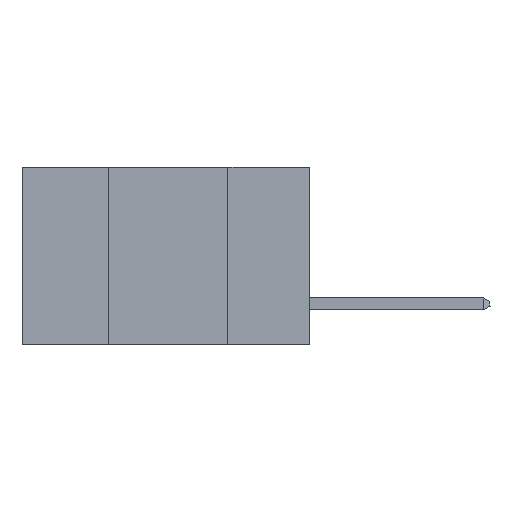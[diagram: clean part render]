
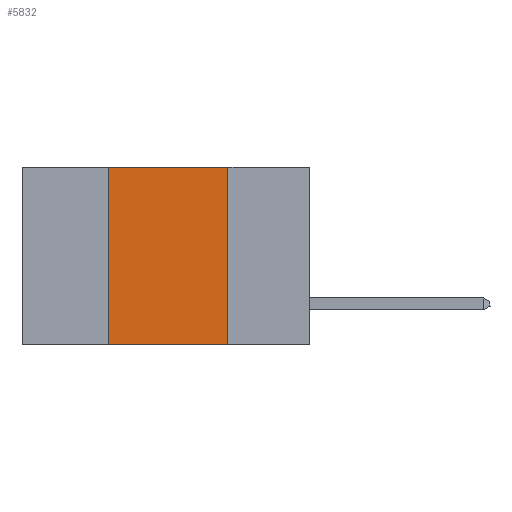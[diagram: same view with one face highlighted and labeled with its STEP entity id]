
A CAD part, left-side view. The second image highlights one B-rep face of the part: STEP entity #5832.
In plain terms, the highlighted planar face has unit normal (-1, 0, 0).
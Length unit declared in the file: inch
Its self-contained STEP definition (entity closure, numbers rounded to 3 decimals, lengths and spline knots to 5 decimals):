
#355 = DIRECTION ( 'NONE',  ( 0., -1., 0. ) ) ;
#1837 = DIRECTION ( 'NONE',  ( 0., -1., 0. ) ) ;
#2146 = ORIENTED_EDGE ( 'NONE', *, *, #18945, .F. ) ;
#2621 = VERTEX_POINT ( 'NONE', #10807 ) ;
#4374 = LINE ( 'NONE', #6501, #4651 ) ;
#4651 = VECTOR ( 'NONE', #21407, 39.37008 ) ;
#5076 = VERTEX_POINT ( 'NONE', #5207 ) ;
#5207 = CARTESIAN_POINT ( 'NONE',  ( 0., 0.42, 0. ) ) ;
#5384 = VECTOR ( 'NONE', #1837, 39.37008 ) ;
#5832 = ADVANCED_FACE ( 'NONE', ( #17424 ), #8938, .F. ) ;
#6370 = EDGE_CURVE ( 'NONE', #14879, #2621, #12262, .T. ) ;
#6501 = CARTESIAN_POINT ( 'NONE',  ( 0., 0.17, 0. ) ) ;
#7292 = CARTESIAN_POINT ( 'NONE',  ( 0., 0.42, 0. ) ) ;
#7399 = CARTESIAN_POINT ( 'NONE',  ( 0., 0.6, 0. ) ) ;
#7805 = EDGE_CURVE ( 'NONE', #16704, #2621, #4374, .T. ) ;
#8421 = LINE ( 'NONE', #7292, #16571 ) ;
#8685 = LINE ( 'NONE', #22218, #18203 ) ;
#8938 = PLANE ( 'NONE',  #21732 ) ;
#10503 = CARTESIAN_POINT ( 'NONE',  ( 0., 0.6, -0.37 ) ) ;
#10643 = DIRECTION ( 'NONE',  ( 0., 0., -1. ) ) ;
#10807 = CARTESIAN_POINT ( 'NONE',  ( 0., 0.17, -0.37 ) ) ;
#11539 = CARTESIAN_POINT ( 'NONE',  ( 0., 0.42, -0.37 ) ) ;
#11978 = EDGE_LOOP ( 'NONE', ( #21581, #2146, #12144, #13847 ) ) ;
#12144 = ORIENTED_EDGE ( 'NONE', *, *, #21015, .F. ) ;
#12262 = LINE ( 'NONE', #10503, #5384 ) ;
#12327 = DIRECTION ( 'NONE',  ( 1., 0., 0. ) ) ;
#13510 = CARTESIAN_POINT ( 'NONE',  ( 0., 0.17, 0. ) ) ;
#13847 = ORIENTED_EDGE ( 'NONE', *, *, #6370, .T. ) ;
#14879 = VERTEX_POINT ( 'NONE', #11539 ) ;
#16571 = VECTOR ( 'NONE', #21004, 39.37008 ) ;
#16704 = VERTEX_POINT ( 'NONE', #13510 ) ;
#17424 = FACE_OUTER_BOUND ( 'NONE', #11978, .T. ) ;
#18203 = VECTOR ( 'NONE', #355, 39.37008 ) ;
#18945 = EDGE_CURVE ( 'NONE', #5076, #16704, #8685, .T. ) ;
#21004 = DIRECTION ( 'NONE',  ( 0., 0., 1. ) ) ;
#21015 = EDGE_CURVE ( 'NONE', #14879, #5076, #8421, .T. ) ;
#21407 = DIRECTION ( 'NONE',  ( 0., 0., -1. ) ) ;
#21581 = ORIENTED_EDGE ( 'NONE', *, *, #7805, .F. ) ;
#21732 = AXIS2_PLACEMENT_3D ( 'NONE', #7399, #12327, #10643 ) ;
#22218 = CARTESIAN_POINT ( 'NONE',  ( 0., 0.6, 0. ) ) ;
